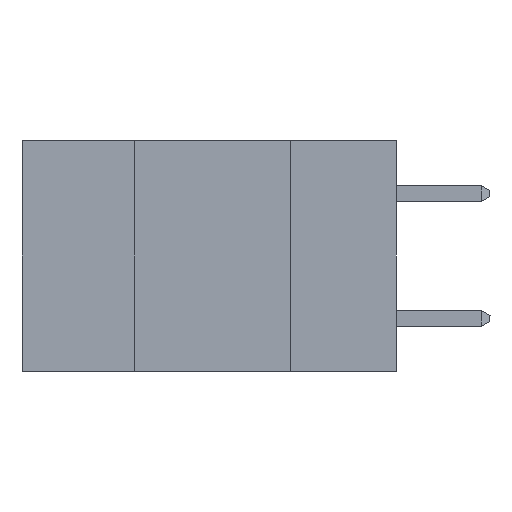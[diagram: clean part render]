
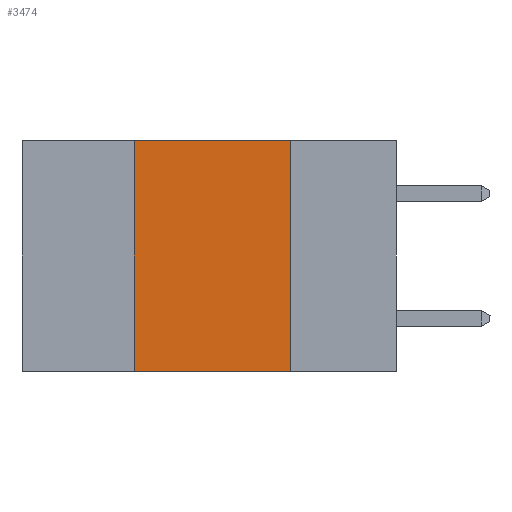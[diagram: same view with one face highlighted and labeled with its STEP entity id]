
A CAD part, left-side view. The second image highlights one B-rep face of the part: STEP entity #3474.
In plain terms, the highlighted planar face has unit normal (-1, 0, 0).
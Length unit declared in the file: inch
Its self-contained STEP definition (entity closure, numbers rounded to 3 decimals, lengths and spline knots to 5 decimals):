
#455 = CARTESIAN_POINT ( 'NONE',  ( 0., 0.6, -0.37 ) ) ;
#471 = PLANE ( 'NONE',  #16830 ) ;
#608 = VECTOR ( 'NONE', #11995, 39.37008 ) ;
#639 = VERTEX_POINT ( 'NONE', #15436 ) ;
#670 = ORIENTED_EDGE ( 'NONE', *, *, #1250, .F. ) ;
#1250 = EDGE_CURVE ( 'NONE', #9781, #639, #4398, .T. ) ;
#1960 = CARTESIAN_POINT ( 'NONE',  ( 0., 0.17, -0.37 ) ) ;
#2104 = DIRECTION ( 'NONE',  ( 1., 0., 0. ) ) ;
#3474 = ADVANCED_FACE ( 'NONE', ( #16778 ), #471, .F. ) ;
#4163 = CARTESIAN_POINT ( 'NONE',  ( 0., 0.17, 0. ) ) ;
#4398 = LINE ( 'NONE', #15200, #608 ) ;
#4690 = VECTOR ( 'NONE', #12571, 39.37008 ) ;
#7437 = EDGE_LOOP ( 'NONE', ( #14413, #10698, #670, #19524 ) ) ;
#9781 = VERTEX_POINT ( 'NONE', #14693 ) ;
#10698 = ORIENTED_EDGE ( 'NONE', *, *, #13920, .F. ) ;
#10992 = CARTESIAN_POINT ( 'NONE',  ( 0., 0.6, 0. ) ) ;
#11231 = EDGE_CURVE ( 'NONE', #20471, #11662, #11819, .T. ) ;
#11631 = CARTESIAN_POINT ( 'NONE',  ( 0., 0.6, 0. ) ) ;
#11662 = VERTEX_POINT ( 'NONE', #1960 ) ;
#11819 = LINE ( 'NONE', #16897, #19829 ) ;
#11995 = DIRECTION ( 'NONE',  ( 0., 0., 1. ) ) ;
#12155 = VECTOR ( 'NONE', #14752, 39.37008 ) ;
#12571 = DIRECTION ( 'NONE',  ( 0., -1., 0. ) ) ;
#12635 = LINE ( 'NONE', #455, #12155 ) ;
#13229 = DIRECTION ( 'NONE',  ( 0., 0., -1. ) ) ;
#13545 = EDGE_CURVE ( 'NONE', #9781, #11662, #12635, .T. ) ;
#13920 = EDGE_CURVE ( 'NONE', #639, #20471, #14131, .T. ) ;
#14131 = LINE ( 'NONE', #10992, #4690 ) ;
#14413 = ORIENTED_EDGE ( 'NONE', *, *, #11231, .F. ) ;
#14693 = CARTESIAN_POINT ( 'NONE',  ( 0., 0.42, -0.37 ) ) ;
#14752 = DIRECTION ( 'NONE',  ( 0., -1., 0. ) ) ;
#15200 = CARTESIAN_POINT ( 'NONE',  ( 0., 0.42, -0.37 ) ) ;
#15436 = CARTESIAN_POINT ( 'NONE',  ( 0., 0.42, 0. ) ) ;
#16778 = FACE_OUTER_BOUND ( 'NONE', #7437, .T. ) ;
#16830 = AXIS2_PLACEMENT_3D ( 'NONE', #11631, #2104, #13229 ) ;
#16897 = CARTESIAN_POINT ( 'NONE',  ( 0., 0.17, -0.37 ) ) ;
#16965 = DIRECTION ( 'NONE',  ( 0., 0., -1. ) ) ;
#19524 = ORIENTED_EDGE ( 'NONE', *, *, #13545, .T. ) ;
#19829 = VECTOR ( 'NONE', #16965, 39.37008 ) ;
#20471 = VERTEX_POINT ( 'NONE', #4163 ) ;
